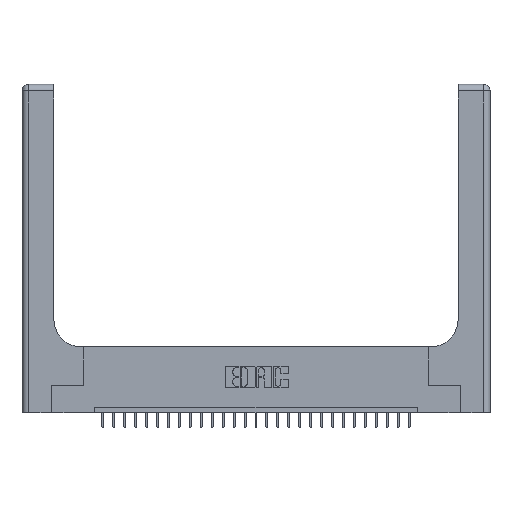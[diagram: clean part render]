
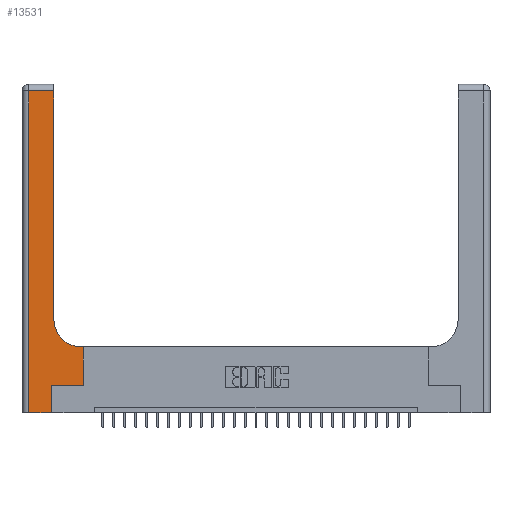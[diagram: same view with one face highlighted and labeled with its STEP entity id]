
A CAD part, top view. The second image highlights one B-rep face of the part: STEP entity #13531.
In plain terms, the highlighted planar face has unit normal (0, 0, 1).
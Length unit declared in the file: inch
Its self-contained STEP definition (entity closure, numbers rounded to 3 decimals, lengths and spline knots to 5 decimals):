
#1002 = VECTOR ( 'NONE', #14961, 39.37008 ) ;
#1269 = PLANE ( 'NONE',  #21245 ) ;
#2001 = CARTESIAN_POINT ( 'NONE',  ( 0.269, 0.25, 0.37 ) ) ;
#2570 = CARTESIAN_POINT ( 'NONE',  ( 0.5585, 0.25, 0.37 ) ) ;
#2710 = DIRECTION ( 'NONE',  ( 0., 1., 0. ) ) ;
#3104 = ORIENTED_EDGE ( 'NONE', *, *, #7754, .T. ) ;
#3123 = VERTEX_POINT ( 'NONE', #13397 ) ;
#3363 = ORIENTED_EDGE ( 'NONE', *, *, #14810, .T. ) ;
#4245 = CARTESIAN_POINT ( 'NONE',  ( 0., 2.94, 0.37 ) ) ;
#4336 = VERTEX_POINT ( 'NONE', #2001 ) ;
#4659 = DIRECTION ( 'NONE',  ( 1., 0., 0. ) ) ;
#5400 = DIRECTION ( 'NONE',  ( 1., 0., 0. ) ) ;
#5406 = EDGE_CURVE ( 'NONE', #4336, #3123, #20610, .T. ) ;
#5485 = CARTESIAN_POINT ( 'NONE',  ( 0.2915, 2.94, 0.37 ) ) ;
#5804 = CARTESIAN_POINT ( 'NONE',  ( 0., 3., 0.37 ) ) ;
#5925 = AXIS2_PLACEMENT_3D ( 'NONE', #7592, #16525, #5400 ) ;
#6151 = CARTESIAN_POINT ( 'NONE',  ( 0., 0., 0.37 ) ) ;
#6201 = ORIENTED_EDGE ( 'NONE', *, *, #27435, .T. ) ;
#6554 = DIRECTION ( 'NONE',  ( -1., 0., 0. ) ) ;
#7204 = EDGE_LOOP ( 'NONE', ( #11755, #6201, #13453, #3104, #22780, #11132, #26335, #16029, #3363 ) ) ;
#7536 = VERTEX_POINT ( 'NONE', #15687 ) ;
#7592 = CARTESIAN_POINT ( 'NONE',  ( 0.5415, 0.85, 0.37 ) ) ;
#7754 = EDGE_CURVE ( 'NONE', #13816, #16084, #10987, .T. ) ;
#8272 = EDGE_CURVE ( 'NONE', #18460, #18344, #22474, .T. ) ;
#8342 = LINE ( 'NONE', #4245, #16096 ) ;
#8490 = DIRECTION ( 'NONE',  ( -1., 0., 0. ) ) ;
#8747 = CARTESIAN_POINT ( 'NONE',  ( 0.2915, 0.6, 0.37 ) ) ;
#10196 = DIRECTION ( 'NONE',  ( 0., 0., -1. ) ) ;
#10554 = DIRECTION ( 'NONE',  ( 1., 0., 0. ) ) ;
#10987 = LINE ( 'NONE', #6151, #22463 ) ;
#11132 = ORIENTED_EDGE ( 'NONE', *, *, #5406, .T. ) ;
#11755 = ORIENTED_EDGE ( 'NONE', *, *, #23045, .T. ) ;
#11942 = VECTOR ( 'NONE', #2710, 39.37008 ) ;
#13146 = CARTESIAN_POINT ( 'NONE',  ( 0.5585, 0.6, 0.37 ) ) ;
#13182 = VECTOR ( 'NONE', #6554, 39.37008 ) ;
#13254 = CARTESIAN_POINT ( 'NONE',  ( 0.06, 3., 0.37 ) ) ;
#13397 = CARTESIAN_POINT ( 'NONE',  ( 0.5585, 0.25, 0.37 ) ) ;
#13453 = ORIENTED_EDGE ( 'NONE', *, *, #19023, .T. ) ;
#13531 = ADVANCED_FACE ( 'NONE', ( #23486 ), #1269, .F. ) ;
#13816 = VERTEX_POINT ( 'NONE', #23297 ) ;
#14127 = LINE ( 'NONE', #2570, #11942 ) ;
#14810 = EDGE_CURVE ( 'NONE', #18344, #7536, #23657, .T. ) ;
#14814 = CARTESIAN_POINT ( 'NONE',  ( 0.2915, 3., 0.37 ) ) ;
#14961 = DIRECTION ( 'NONE',  ( 0., 1., 0. ) ) ;
#15440 = LINE ( 'NONE', #13254, #19602 ) ;
#15476 = DIRECTION ( 'NONE',  ( 0., 1., 0. ) ) ;
#15581 = DIRECTION ( 'NONE',  ( 0., -1., 0. ) ) ;
#15687 = CARTESIAN_POINT ( 'NONE',  ( 0.2915, 0.85, 0.37 ) ) ;
#16029 = ORIENTED_EDGE ( 'NONE', *, *, #8272, .T. ) ;
#16084 = VERTEX_POINT ( 'NONE', #20166 ) ;
#16096 = VECTOR ( 'NONE', #8490, 39.37008 ) ;
#16368 = CARTESIAN_POINT ( 'NONE',  ( 0.269, 0.25, 0.37 ) ) ;
#16525 = DIRECTION ( 'NONE',  ( 0., 0., -1. ) ) ;
#17484 = EDGE_CURVE ( 'NONE', #16084, #4336, #20569, .T. ) ;
#17598 = VERTEX_POINT ( 'NONE', #5485 ) ;
#17795 = CARTESIAN_POINT ( 'NONE',  ( 0.269, 0., 0.37 ) ) ;
#18344 = VERTEX_POINT ( 'NONE', #23363 ) ;
#18460 = VERTEX_POINT ( 'NONE', #13146 ) ;
#19023 = EDGE_CURVE ( 'NONE', #19417, #13816, #15440, .T. ) ;
#19111 = DIRECTION ( 'NONE',  ( -1., 0., 0. ) ) ;
#19417 = VERTEX_POINT ( 'NONE', #22242 ) ;
#19602 = VECTOR ( 'NONE', #15581, 39.37008 ) ;
#19997 = VECTOR ( 'NONE', #15476, 39.37008 ) ;
#20166 = CARTESIAN_POINT ( 'NONE',  ( 0.269, 0., 0.37 ) ) ;
#20569 = LINE ( 'NONE', #17795, #19997 ) ;
#20610 = LINE ( 'NONE', #16368, #24215 ) ;
#21245 = AXIS2_PLACEMENT_3D ( 'NONE', #5804, #10196, #19111 ) ;
#22242 = CARTESIAN_POINT ( 'NONE',  ( 0.06, 2.94, 0.37 ) ) ;
#22463 = VECTOR ( 'NONE', #10554, 39.37008 ) ;
#22474 = LINE ( 'NONE', #8747, #13182 ) ;
#22780 = ORIENTED_EDGE ( 'NONE', *, *, #17484, .T. ) ;
#23045 = EDGE_CURVE ( 'NONE', #7536, #17598, #28213, .T. ) ;
#23297 = CARTESIAN_POINT ( 'NONE',  ( 0.06, 0., 0.37 ) ) ;
#23363 = CARTESIAN_POINT ( 'NONE',  ( 0.5415, 0.6, 0.37 ) ) ;
#23486 = FACE_OUTER_BOUND ( 'NONE', #7204, .T. ) ;
#23657 = CIRCLE ( 'NONE', #5925, 0.25 ) ;
#24215 = VECTOR ( 'NONE', #4659, 39.37008 ) ;
#26335 = ORIENTED_EDGE ( 'NONE', *, *, #28085, .T. ) ;
#27435 = EDGE_CURVE ( 'NONE', #17598, #19417, #8342, .T. ) ;
#28085 = EDGE_CURVE ( 'NONE', #3123, #18460, #14127, .T. ) ;
#28213 = LINE ( 'NONE', #14814, #1002 ) ;
